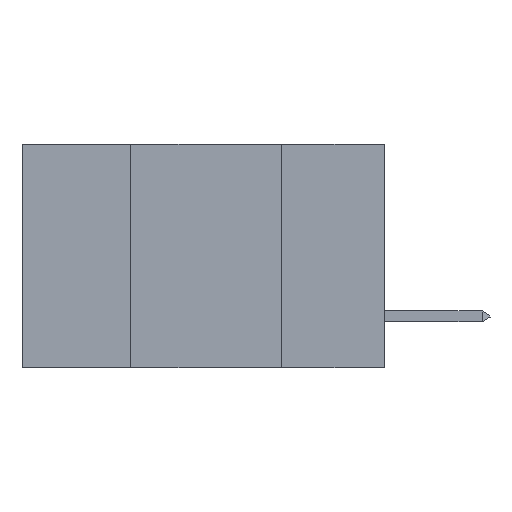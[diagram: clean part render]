
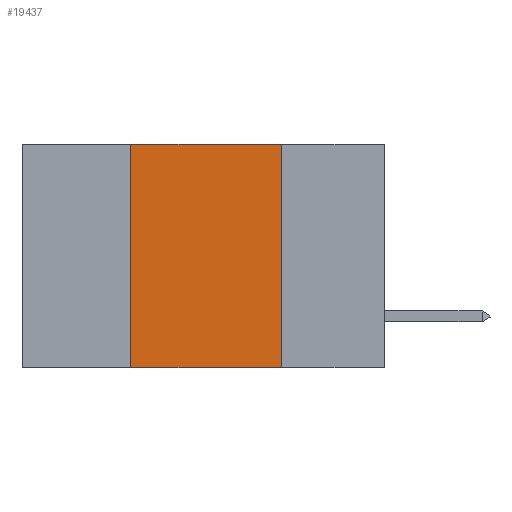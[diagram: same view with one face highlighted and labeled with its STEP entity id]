
A CAD part, left-side view. The second image highlights one B-rep face of the part: STEP entity #19437.
In plain terms, the highlighted planar face has unit normal (-1, 0, 0).
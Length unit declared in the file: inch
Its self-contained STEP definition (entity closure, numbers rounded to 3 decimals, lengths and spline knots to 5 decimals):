
#627 = DIRECTION ( 'NONE',  ( 1., 0., 0. ) ) ;
#721 = CARTESIAN_POINT ( 'NONE',  ( 0., 0.6, -0.37 ) ) ;
#782 = EDGE_CURVE ( 'NONE', #8643, #19083, #10879, .T. ) ;
#1479 = ORIENTED_EDGE ( 'NONE', *, *, #782, .F. ) ;
#1789 = ORIENTED_EDGE ( 'NONE', *, *, #20598, .F. ) ;
#3520 = CARTESIAN_POINT ( 'NONE',  ( 0., 0.17, 0. ) ) ;
#4630 = CARTESIAN_POINT ( 'NONE',  ( 0., 0.42, 0. ) ) ;
#4729 = CARTESIAN_POINT ( 'NONE',  ( 0., 0.42, -0.37 ) ) ;
#6837 = LINE ( 'NONE', #10954, #15587 ) ;
#6863 = CARTESIAN_POINT ( 'NONE',  ( 0., 0.17, 0. ) ) ;
#7864 = PLANE ( 'NONE',  #20750 ) ;
#8640 = DIRECTION ( 'NONE',  ( 0., 0., -1. ) ) ;
#8643 = VERTEX_POINT ( 'NONE', #3520 ) ;
#9268 = LINE ( 'NONE', #721, #19068 ) ;
#10212 = EDGE_LOOP ( 'NONE', ( #1479, #17249, #1789, #18311 ) ) ;
#10449 = VERTEX_POINT ( 'NONE', #4630 ) ;
#10560 = EDGE_CURVE ( 'NONE', #10449, #8643, #6837, .T. ) ;
#10850 = DIRECTION ( 'NONE',  ( 0., 0., 1. ) ) ;
#10879 = LINE ( 'NONE', #6863, #14161 ) ;
#10954 = CARTESIAN_POINT ( 'NONE',  ( 0., 0.6, 0. ) ) ;
#11704 = EDGE_CURVE ( 'NONE', #18233, #19083, #9268, .T. ) ;
#12399 = CARTESIAN_POINT ( 'NONE',  ( 0., 0.17, -0.37 ) ) ;
#14161 = VECTOR ( 'NONE', #8640, 39.37008 ) ;
#14232 = DIRECTION ( 'NONE',  ( 0., -1., 0. ) ) ;
#14611 = VECTOR ( 'NONE', #10850, 39.37008 ) ;
#14745 = CARTESIAN_POINT ( 'NONE',  ( 0., 0.6, 0. ) ) ;
#15587 = VECTOR ( 'NONE', #14232, 39.37008 ) ;
#17249 = ORIENTED_EDGE ( 'NONE', *, *, #10560, .F. ) ;
#18009 = CARTESIAN_POINT ( 'NONE',  ( 0., 0.42, 0. ) ) ;
#18114 = DIRECTION ( 'NONE',  ( 0., -1., 0. ) ) ;
#18233 = VERTEX_POINT ( 'NONE', #4729 ) ;
#18311 = ORIENTED_EDGE ( 'NONE', *, *, #11704, .T. ) ;
#18740 = FACE_OUTER_BOUND ( 'NONE', #10212, .T. ) ;
#19068 = VECTOR ( 'NONE', #18114, 39.37008 ) ;
#19083 = VERTEX_POINT ( 'NONE', #12399 ) ;
#19437 = ADVANCED_FACE ( 'NONE', ( #18740 ), #7864, .F. ) ;
#20061 = DIRECTION ( 'NONE',  ( 0., 0., -1. ) ) ;
#20318 = LINE ( 'NONE', #18009, #14611 ) ;
#20598 = EDGE_CURVE ( 'NONE', #18233, #10449, #20318, .T. ) ;
#20750 = AXIS2_PLACEMENT_3D ( 'NONE', #14745, #627, #20061 ) ;
